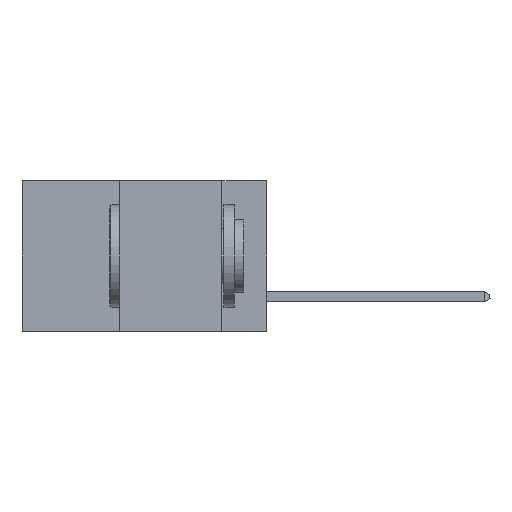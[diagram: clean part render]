
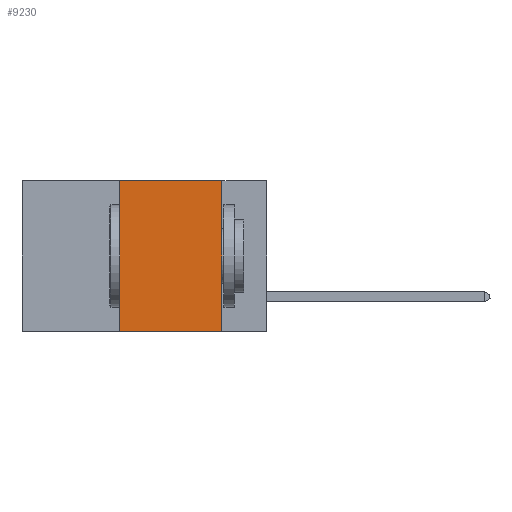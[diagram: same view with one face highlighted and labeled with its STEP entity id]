
A CAD part, left-side view. The second image highlights one B-rep face of the part: STEP entity #9230.
In plain terms, the highlighted planar face has unit normal (-1, 0, 0).
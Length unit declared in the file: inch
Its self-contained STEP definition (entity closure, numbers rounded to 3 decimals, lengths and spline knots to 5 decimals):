
#715 = CARTESIAN_POINT ( 'NONE',  ( 0., 0.6, -0.37 ) ) ;
#2545 = LINE ( 'NONE', #25181, #2869 ) ;
#2750 = VECTOR ( 'NONE', #9502, 39.37008 ) ;
#2869 = VECTOR ( 'NONE', #2932, 39.37008 ) ;
#2919 = DIRECTION ( 'NONE',  ( 0., -1., 0. ) ) ;
#2932 = DIRECTION ( 'NONE',  ( 0., 0., -1. ) ) ;
#3011 = VERTEX_POINT ( 'NONE', #13090 ) ;
#3413 = CARTESIAN_POINT ( 'NONE',  ( 0., 0.11, -0.37 ) ) ;
#5462 = ORIENTED_EDGE ( 'NONE', *, *, #8096, .F. ) ;
#5478 = CARTESIAN_POINT ( 'NONE',  ( 0., 0.6, 0. ) ) ;
#6764 = CARTESIAN_POINT ( 'NONE',  ( 0., 0.36, 0. ) ) ;
#7796 = VECTOR ( 'NONE', #2919, 39.37008 ) ;
#8096 = EDGE_CURVE ( 'NONE', #23258, #25290, #15015, .T. ) ;
#9230 = ADVANCED_FACE ( 'NONE', ( #11128 ), #18459, .F. ) ;
#9274 = ORIENTED_EDGE ( 'NONE', *, *, #25304, .F. ) ;
#9502 = DIRECTION ( 'NONE',  ( 0., -1., 0. ) ) ;
#11128 = FACE_OUTER_BOUND ( 'NONE', #23497, .T. ) ;
#11577 = LINE ( 'NONE', #715, #7796 ) ;
#12182 = EDGE_CURVE ( 'NONE', #23258, #20732, #11577, .T. ) ;
#12216 = AXIS2_PLACEMENT_3D ( 'NONE', #26179, #14017, #16036 ) ;
#13090 = CARTESIAN_POINT ( 'NONE',  ( 0., 0.11, 0. ) ) ;
#14017 = DIRECTION ( 'NONE',  ( 1., 0., 0. ) ) ;
#14889 = DIRECTION ( 'NONE',  ( 0., 0., 1. ) ) ;
#15015 = LINE ( 'NONE', #6764, #25838 ) ;
#16036 = DIRECTION ( 'NONE',  ( 0., 0., -1. ) ) ;
#17632 = ORIENTED_EDGE ( 'NONE', *, *, #23336, .F. ) ;
#18459 = PLANE ( 'NONE',  #12216 ) ;
#18604 = LINE ( 'NONE', #5478, #2750 ) ;
#20732 = VERTEX_POINT ( 'NONE', #3413 ) ;
#21063 = CARTESIAN_POINT ( 'NONE',  ( 0., 0.36, -0.37 ) ) ;
#21636 = CARTESIAN_POINT ( 'NONE',  ( 0., 0.36, 0. ) ) ;
#23258 = VERTEX_POINT ( 'NONE', #21063 ) ;
#23336 = EDGE_CURVE ( 'NONE', #3011, #20732, #2545, .T. ) ;
#23497 = EDGE_LOOP ( 'NONE', ( #17632, #9274, #5462, #25305 ) ) ;
#25181 = CARTESIAN_POINT ( 'NONE',  ( 0., 0.11, 0. ) ) ;
#25290 = VERTEX_POINT ( 'NONE', #21636 ) ;
#25304 = EDGE_CURVE ( 'NONE', #25290, #3011, #18604, .T. ) ;
#25305 = ORIENTED_EDGE ( 'NONE', *, *, #12182, .T. ) ;
#25838 = VECTOR ( 'NONE', #14889, 39.37008 ) ;
#26179 = CARTESIAN_POINT ( 'NONE',  ( 0., 0.6, 0. ) ) ;
